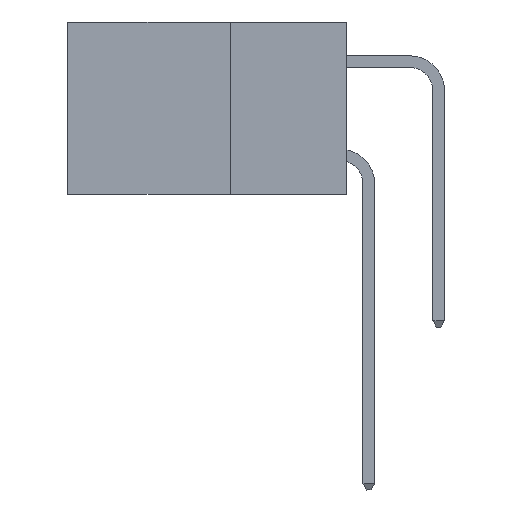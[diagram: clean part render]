
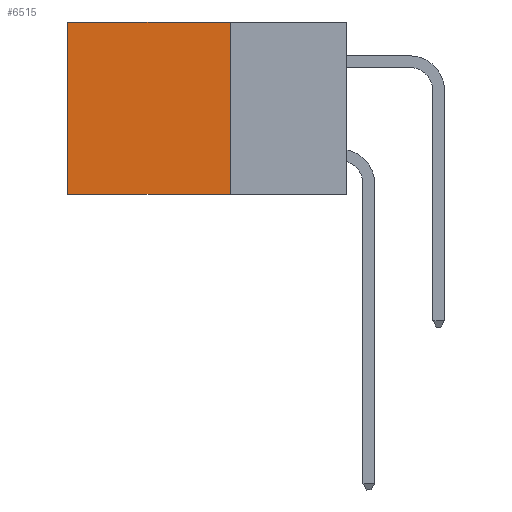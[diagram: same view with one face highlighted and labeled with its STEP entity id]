
A CAD part, left-side view. The second image highlights one B-rep face of the part: STEP entity #6515.
In plain terms, the highlighted planar face has unit normal (-1, 0, 0).
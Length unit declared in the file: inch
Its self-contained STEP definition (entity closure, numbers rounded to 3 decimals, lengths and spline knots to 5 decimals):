
#346 = DIRECTION ( 'NONE',  ( 1., 0., 0. ) ) ;
#512 = DIRECTION ( 'NONE',  ( 0., 1., 0. ) ) ;
#535 = VERTEX_POINT ( 'NONE', #13963 ) ;
#694 = LINE ( 'NONE', #13954, #6758 ) ;
#1159 = ORIENTED_EDGE ( 'NONE', *, *, #12871, .F. ) ;
#1595 = CARTESIAN_POINT ( 'NONE',  ( 0.2875, 0.6, 0. ) ) ;
#3933 = PLANE ( 'NONE',  #10453 ) ;
#4048 = DIRECTION ( 'NONE',  ( 0., 0., -1. ) ) ;
#4601 = FACE_OUTER_BOUND ( 'NONE', #6664, .T. ) ;
#4912 = DIRECTION ( 'NONE',  ( 0., 1., 0. ) ) ;
#5129 = EDGE_CURVE ( 'NONE', #7953, #5749, #694, .T. ) ;
#5159 = ORIENTED_EDGE ( 'NONE', *, *, #10441, .F. ) ;
#5749 = VERTEX_POINT ( 'NONE', #13881 ) ;
#6166 = CARTESIAN_POINT ( 'NONE',  ( 0.2875, 0.25, 0. ) ) ;
#6378 = CARTESIAN_POINT ( 'NONE',  ( 0.2875, 0.25, 0. ) ) ;
#6515 = ADVANCED_FACE ( 'NONE', ( #4601 ), #3933, .F. ) ;
#6664 = EDGE_LOOP ( 'NONE', ( #6853, #1159, #5159, #11350 ) ) ;
#6758 = VECTOR ( 'NONE', #512, 39.37008 ) ;
#6853 = ORIENTED_EDGE ( 'NONE', *, *, #10626, .T. ) ;
#7345 = DIRECTION ( 'NONE',  ( 0., 0., -1. ) ) ;
#7953 = VERTEX_POINT ( 'NONE', #10678 ) ;
#8032 = LINE ( 'NONE', #6166, #13271 ) ;
#8185 = LINE ( 'NONE', #11511, #13423 ) ;
#8613 = DIRECTION ( 'NONE',  ( 0., 0., -1. ) ) ;
#10441 = EDGE_CURVE ( 'NONE', #7953, #14188, #8032, .T. ) ;
#10453 = AXIS2_PLACEMENT_3D ( 'NONE', #6378, #346, #8613 ) ;
#10626 = EDGE_CURVE ( 'NONE', #5749, #535, #14061, .T. ) ;
#10678 = CARTESIAN_POINT ( 'NONE',  ( 0.2875, 0.25, 0. ) ) ;
#11300 = VECTOR ( 'NONE', #4048, 39.37008 ) ;
#11350 = ORIENTED_EDGE ( 'NONE', *, *, #5129, .T. ) ;
#11511 = CARTESIAN_POINT ( 'NONE',  ( 0.2875, 0.25, -0.37 ) ) ;
#12871 = EDGE_CURVE ( 'NONE', #14188, #535, #8185, .T. ) ;
#13144 = CARTESIAN_POINT ( 'NONE',  ( 0.2875, 0.25, -0.37 ) ) ;
#13271 = VECTOR ( 'NONE', #7345, 39.37008 ) ;
#13423 = VECTOR ( 'NONE', #4912, 39.37008 ) ;
#13881 = CARTESIAN_POINT ( 'NONE',  ( 0.2875, 0.6, 0. ) ) ;
#13954 = CARTESIAN_POINT ( 'NONE',  ( 0.2875, 0.25, 0. ) ) ;
#13963 = CARTESIAN_POINT ( 'NONE',  ( 0.2875, 0.6, -0.37 ) ) ;
#14061 = LINE ( 'NONE', #1595, #11300 ) ;
#14188 = VERTEX_POINT ( 'NONE', #13144 ) ;
